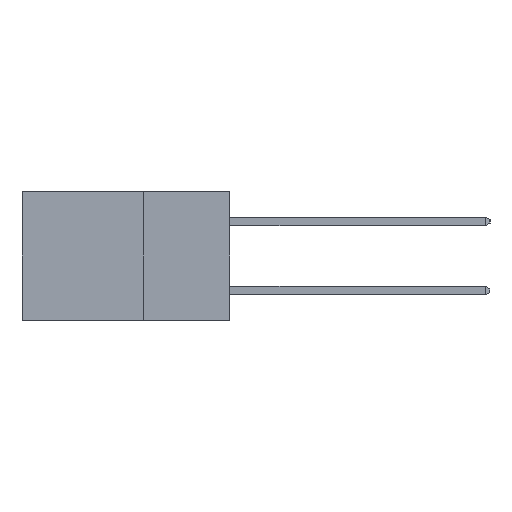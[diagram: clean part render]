
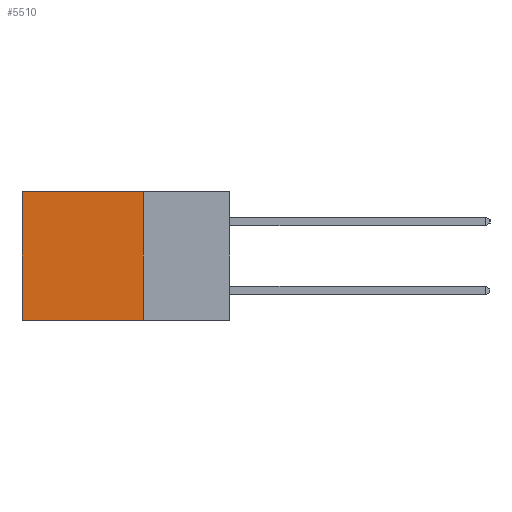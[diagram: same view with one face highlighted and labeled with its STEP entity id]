
A CAD part, left-side view. The second image highlights one B-rep face of the part: STEP entity #5510.
In plain terms, the highlighted planar face has unit normal (-1, 0, 0).
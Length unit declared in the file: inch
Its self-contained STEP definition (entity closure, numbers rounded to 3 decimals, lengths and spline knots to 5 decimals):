
#43 = EDGE_CURVE ( 'NONE', #380, #21786, #17292, .T. ) ;
#380 = VERTEX_POINT ( 'NONE', #26215 ) ;
#2634 = CARTESIAN_POINT ( 'NONE',  ( 0.298, 0.6, -0.37 ) ) ;
#4039 = CARTESIAN_POINT ( 'NONE',  ( 0.298, 0.25, 0. ) ) ;
#4350 = VECTOR ( 'NONE', #24134, 39.37008 ) ;
#4980 = LINE ( 'NONE', #26168, #4350 ) ;
#5510 = ADVANCED_FACE ( 'NONE', ( #12731 ), #17813, .F. ) ;
#6316 = ORIENTED_EDGE ( 'NONE', *, *, #14645, .F. ) ;
#6562 = DIRECTION ( 'NONE',  ( 0., 1., 0. ) ) ;
#7310 = ORIENTED_EDGE ( 'NONE', *, *, #10308, .F. ) ;
#8428 = LINE ( 'NONE', #26159, #19013 ) ;
#9308 = EDGE_LOOP ( 'NONE', ( #19855, #7310, #6316, #24256 ) ) ;
#10308 = EDGE_CURVE ( 'NONE', #10809, #21786, #10996, .T. ) ;
#10523 = CARTESIAN_POINT ( 'NONE',  ( 0.298, 0.25, 0. ) ) ;
#10809 = VERTEX_POINT ( 'NONE', #22853 ) ;
#10996 = LINE ( 'NONE', #17050, #21567 ) ;
#11190 = DIRECTION ( 'NONE',  ( 0., 0., -1. ) ) ;
#12165 = VERTEX_POINT ( 'NONE', #10523 ) ;
#12731 = FACE_OUTER_BOUND ( 'NONE', #9308, .T. ) ;
#14645 = EDGE_CURVE ( 'NONE', #12165, #10809, #8428, .T. ) ;
#16525 = DIRECTION ( 'NONE',  ( 0., 0., -1. ) ) ;
#17050 = CARTESIAN_POINT ( 'NONE',  ( 0.298, 0.25, -0.37 ) ) ;
#17292 = LINE ( 'NONE', #21023, #22923 ) ;
#17479 = DIRECTION ( 'NONE',  ( 1., 0., 0. ) ) ;
#17768 = DIRECTION ( 'NONE',  ( 0., 0., -1. ) ) ;
#17813 = PLANE ( 'NONE',  #18381 ) ;
#18381 = AXIS2_PLACEMENT_3D ( 'NONE', #4039, #17479, #11190 ) ;
#19013 = VECTOR ( 'NONE', #17768, 39.37008 ) ;
#19855 = ORIENTED_EDGE ( 'NONE', *, *, #43, .T. ) ;
#20556 = EDGE_CURVE ( 'NONE', #12165, #380, #4980, .T. ) ;
#21023 = CARTESIAN_POINT ( 'NONE',  ( 0.298, 0.6, 0. ) ) ;
#21567 = VECTOR ( 'NONE', #6562, 39.37008 ) ;
#21786 = VERTEX_POINT ( 'NONE', #2634 ) ;
#22853 = CARTESIAN_POINT ( 'NONE',  ( 0.298, 0.25, -0.37 ) ) ;
#22923 = VECTOR ( 'NONE', #16525, 39.37008 ) ;
#24134 = DIRECTION ( 'NONE',  ( 0., 1., 0. ) ) ;
#24256 = ORIENTED_EDGE ( 'NONE', *, *, #20556, .T. ) ;
#26159 = CARTESIAN_POINT ( 'NONE',  ( 0.298, 0.25, 0. ) ) ;
#26168 = CARTESIAN_POINT ( 'NONE',  ( 0.298, 0.25, 0. ) ) ;
#26215 = CARTESIAN_POINT ( 'NONE',  ( 0.298, 0.6, 0. ) ) ;
